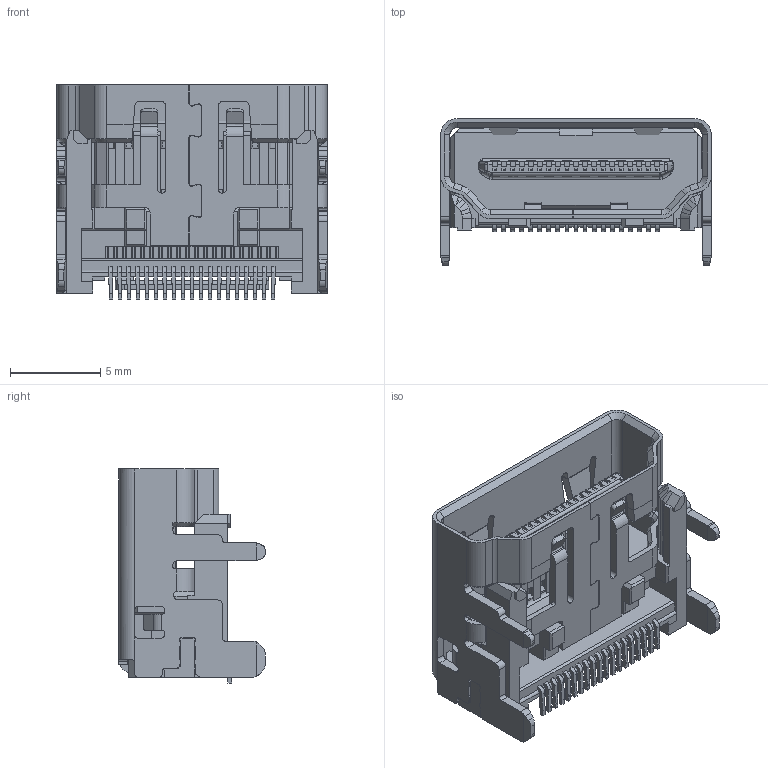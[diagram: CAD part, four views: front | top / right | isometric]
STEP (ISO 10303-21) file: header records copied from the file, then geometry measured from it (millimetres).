
FILE_DESCRIPTION (( 'STEP AP214' ), '1' );
FILE_NAME ('694D119-164-011.STEP', '2021-01-13T15:57:48', ( '' ), ( '' ), 'SwSTEP 2.0', 'SolidWorks 2020', '' );
FILE_SCHEMA (( 'AUTOMOTIVE_DESIGN' ));
Length unit declared in the file: millimetre
Products named in the file (3): Shell 694D119-X64-011; 694D119-164-011; Insulator 694D119-X64-011
Assembly tree (2 placements, depth 2):
  694D119-164-011
    Insulator 694D119-X64-011
    Shell 694D119-X64-011
Bounding box: 15 x 8.13 x 11.87 mm (x, y, z)
Volume: 455.6 mm3; surface area: 1545.7 mm2
Topology: 2 solids, 2 shells, 1880 faces, 5296 edges, 3420 vertices
Faces by surface type: plane 1391, cylinder 429, bspline 32, cone 26, torus 2
Entity records: 65269 total; most frequent: CARTESIAN_POINT 12286, ORIENTED_EDGE 10572, DIRECTION 9409, EDGE_CURVE 5286, LINE 4177, VECTOR 4177, VERTEX_POINT 3420, AXIS2_PLACEMENT_3D 2616
